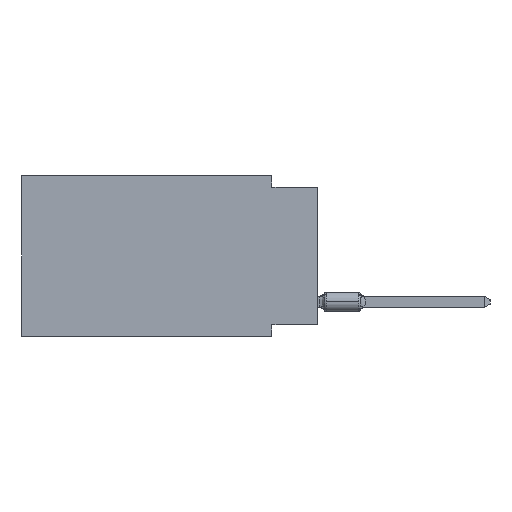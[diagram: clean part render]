
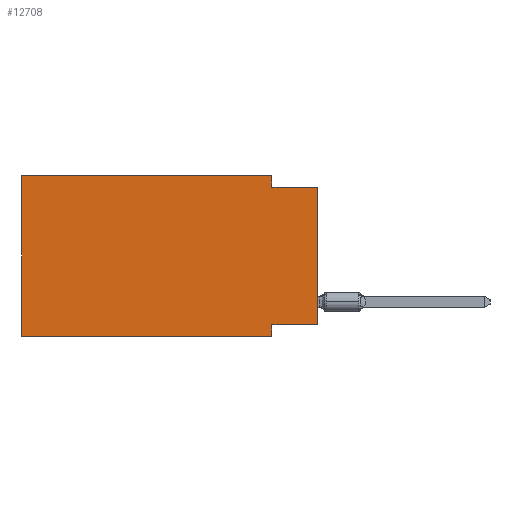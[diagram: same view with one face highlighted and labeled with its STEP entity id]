
A CAD part, left-side view. The second image highlights one B-rep face of the part: STEP entity #12708.
In plain terms, the highlighted planar face has unit normal (-1, 0, 0).
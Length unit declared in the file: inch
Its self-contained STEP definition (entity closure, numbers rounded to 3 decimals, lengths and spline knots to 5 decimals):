
#405 = ORIENTED_EDGE ( 'NONE', *, *, #26666, .F. ) ;
#734 = DIRECTION ( 'NONE',  ( 0., 0., 1. ) ) ;
#1043 = DIRECTION ( 'NONE',  ( 0., -1., 0. ) ) ;
#3159 = CARTESIAN_POINT ( 'NONE',  ( 0., 0., -0.325 ) ) ;
#3920 = VERTEX_POINT ( 'NONE', #20329 ) ;
#4222 = VERTEX_POINT ( 'NONE', #26580 ) ;
#4619 = DIRECTION ( 'NONE',  ( 0., -1., 0. ) ) ;
#4926 = VERTEX_POINT ( 'NONE', #25581 ) ;
#5062 = LINE ( 'NONE', #38426, #42910 ) ;
#6685 = LINE ( 'NONE', #47168, #37846 ) ;
#6737 = EDGE_LOOP ( 'NONE', ( #10612, #28175, #37044, #405, #24923, #33044, #19569, #22014 ) ) ;
#6832 = CARTESIAN_POINT ( 'NONE',  ( 0., 0.645, 0. ) ) ;
#7667 = CARTESIAN_POINT ( 'NONE',  ( 0., 0.1, -0.35 ) ) ;
#9396 = EDGE_CURVE ( 'NONE', #3920, #4926, #39793, .T. ) ;
#9958 = CARTESIAN_POINT ( 'NONE',  ( 0., 0.645, 0. ) ) ;
#10043 = VECTOR ( 'NONE', #22978, 39.37008 ) ;
#10612 = ORIENTED_EDGE ( 'NONE', *, *, #24700, .T. ) ;
#10833 = CARTESIAN_POINT ( 'NONE',  ( 0., 0.1, -0.325 ) ) ;
#10934 = CARTESIAN_POINT ( 'NONE',  ( 0., 0.645, 0. ) ) ;
#11457 = VECTOR ( 'NONE', #1043, 39.37008 ) ;
#12708 = ADVANCED_FACE ( 'NONE', ( #31550 ), #48141, .F. ) ;
#13497 = VERTEX_POINT ( 'NONE', #6832 ) ;
#14670 = CARTESIAN_POINT ( 'NONE',  ( 0., 0., -0.025 ) ) ;
#14724 = CARTESIAN_POINT ( 'NONE',  ( 0., 0., -0.325 ) ) ;
#15112 = VECTOR ( 'NONE', #53307, 39.37008 ) ;
#15479 = VECTOR ( 'NONE', #27055, 39.37008 ) ;
#16034 = LINE ( 'NONE', #38001, #27524 ) ;
#18690 = VERTEX_POINT ( 'NONE', #47892 ) ;
#18886 = VECTOR ( 'NONE', #40603, 39.37008 ) ;
#19569 = ORIENTED_EDGE ( 'NONE', *, *, #43612, .F. ) ;
#20078 = AXIS2_PLACEMENT_3D ( 'NONE', #10934, #25004, #49739 ) ;
#20329 = CARTESIAN_POINT ( 'NONE',  ( 0., 0.1, 0. ) ) ;
#22014 = ORIENTED_EDGE ( 'NONE', *, *, #49454, .F. ) ;
#22978 = DIRECTION ( 'NONE',  ( 0., 0., 1. ) ) ;
#24700 = EDGE_CURVE ( 'NONE', #51359, #29122, #5062, .T. ) ;
#24923 = ORIENTED_EDGE ( 'NONE', *, *, #25410, .F. ) ;
#25004 = DIRECTION ( 'NONE',  ( 1., 0., 0. ) ) ;
#25410 = EDGE_CURVE ( 'NONE', #18690, #13497, #26230, .T. ) ;
#25581 = CARTESIAN_POINT ( 'NONE',  ( 0., 0.1, -0.025 ) ) ;
#26230 = LINE ( 'NONE', #9958, #10043 ) ;
#26580 = CARTESIAN_POINT ( 'NONE',  ( 0., 0.1, -0.35 ) ) ;
#26666 = EDGE_CURVE ( 'NONE', #13497, #3920, #6685, .T. ) ;
#27055 = DIRECTION ( 'NONE',  ( 0., 0., -1. ) ) ;
#27524 = VECTOR ( 'NONE', #4619, 39.37008 ) ;
#28175 = ORIENTED_EDGE ( 'NONE', *, *, #51964, .F. ) ;
#29122 = VERTEX_POINT ( 'NONE', #14670 ) ;
#31550 = FACE_OUTER_BOUND ( 'NONE', #6737, .T. ) ;
#33044 = ORIENTED_EDGE ( 'NONE', *, *, #49093, .T. ) ;
#33882 = LINE ( 'NONE', #37957, #11457 ) ;
#34664 = CARTESIAN_POINT ( 'NONE',  ( 0., 0.1, 0. ) ) ;
#34934 = DIRECTION ( 'NONE',  ( 0., -1., 0. ) ) ;
#36709 = LINE ( 'NONE', #7667, #15112 ) ;
#37044 = ORIENTED_EDGE ( 'NONE', *, *, #9396, .F. ) ;
#37846 = VECTOR ( 'NONE', #34934, 39.37008 ) ;
#37957 = CARTESIAN_POINT ( 'NONE',  ( 0., 0., -0.025 ) ) ;
#38001 = CARTESIAN_POINT ( 'NONE',  ( 0., 0.645, -0.35 ) ) ;
#38426 = CARTESIAN_POINT ( 'NONE',  ( 0., 0., 0. ) ) ;
#39793 = LINE ( 'NONE', #34664, #15479 ) ;
#40603 = DIRECTION ( 'NONE',  ( 0., 1., 0. ) ) ;
#40916 = VERTEX_POINT ( 'NONE', #10833 ) ;
#41131 = LINE ( 'NONE', #3159, #18886 ) ;
#42910 = VECTOR ( 'NONE', #734, 39.37008 ) ;
#43612 = EDGE_CURVE ( 'NONE', #40916, #4222, #36709, .T. ) ;
#47168 = CARTESIAN_POINT ( 'NONE',  ( 0., 0.645, 0. ) ) ;
#47892 = CARTESIAN_POINT ( 'NONE',  ( 0., 0.645, -0.35 ) ) ;
#48141 = PLANE ( 'NONE',  #20078 ) ;
#49093 = EDGE_CURVE ( 'NONE', #18690, #4222, #16034, .T. ) ;
#49454 = EDGE_CURVE ( 'NONE', #51359, #40916, #41131, .T. ) ;
#49739 = DIRECTION ( 'NONE',  ( 0., 0., -1. ) ) ;
#51359 = VERTEX_POINT ( 'NONE', #14724 ) ;
#51964 = EDGE_CURVE ( 'NONE', #4926, #29122, #33882, .T. ) ;
#53307 = DIRECTION ( 'NONE',  ( 0., 0., -1. ) ) ;
